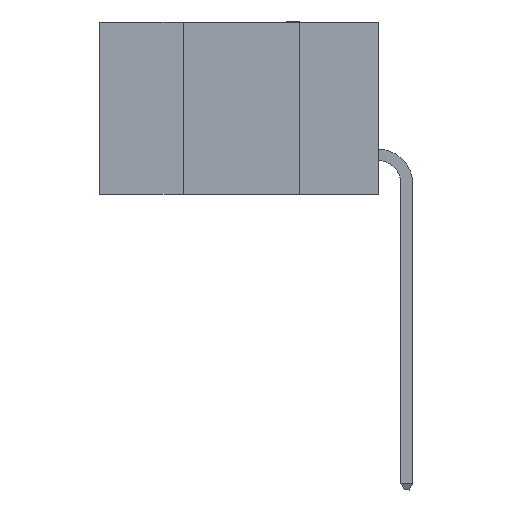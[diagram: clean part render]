
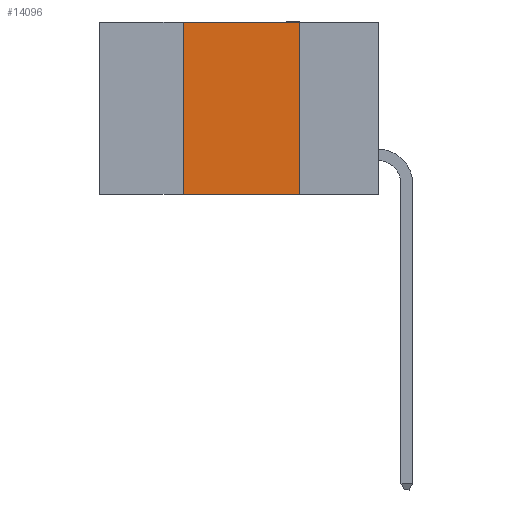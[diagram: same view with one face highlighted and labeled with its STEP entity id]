
A CAD part, left-side view. The second image highlights one B-rep face of the part: STEP entity #14096.
In plain terms, the highlighted planar face has unit normal (-1, 0, 0).
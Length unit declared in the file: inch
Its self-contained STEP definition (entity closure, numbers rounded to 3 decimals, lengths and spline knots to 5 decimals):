
#44 = EDGE_LOOP ( 'NONE', ( #13798, #10727, #9750, #3864 ) ) ;
#393 = FACE_OUTER_BOUND ( 'NONE', #44, .T. ) ;
#962 = VERTEX_POINT ( 'NONE', #5212 ) ;
#1125 = VECTOR ( 'NONE', #3401, 39.37008 ) ;
#1788 = CARTESIAN_POINT ( 'NONE',  ( 0., 0.17, 0. ) ) ;
#1897 = PLANE ( 'NONE',  #8837 ) ;
#2640 = VERTEX_POINT ( 'NONE', #10346 ) ;
#3098 = DIRECTION ( 'NONE',  ( 0., 0., -1. ) ) ;
#3101 = DIRECTION ( 'NONE',  ( 0., 0., 1. ) ) ;
#3401 = DIRECTION ( 'NONE',  ( 0., -1., 0. ) ) ;
#3864 = ORIENTED_EDGE ( 'NONE', *, *, #14314, .T. ) ;
#4632 = VECTOR ( 'NONE', #3101, 39.37008 ) ;
#4751 = DIRECTION ( 'NONE',  ( 0., -1., 0. ) ) ;
#5212 = CARTESIAN_POINT ( 'NONE',  ( 0., 0.17, -0.37 ) ) ;
#5294 = DIRECTION ( 'NONE',  ( 1., 0., 0. ) ) ;
#5387 = CARTESIAN_POINT ( 'NONE',  ( 0., 0.6, 0. ) ) ;
#5408 = LINE ( 'NONE', #10772, #12313 ) ;
#6463 = CARTESIAN_POINT ( 'NONE',  ( 0., 0.17, 0. ) ) ;
#6552 = CARTESIAN_POINT ( 'NONE',  ( 0., 0.42, 0. ) ) ;
#6623 = EDGE_CURVE ( 'NONE', #2640, #13649, #8579, .T. ) ;
#7490 = LINE ( 'NONE', #10611, #1125 ) ;
#8579 = LINE ( 'NONE', #6552, #4632 ) ;
#8610 = EDGE_CURVE ( 'NONE', #15246, #962, #10756, .T. ) ;
#8837 = AXIS2_PLACEMENT_3D ( 'NONE', #5387, #5294, #3098 ) ;
#9067 = CARTESIAN_POINT ( 'NONE',  ( 0., 0.42, 0. ) ) ;
#9750 = ORIENTED_EDGE ( 'NONE', *, *, #6623, .F. ) ;
#9994 = VECTOR ( 'NONE', #12695, 39.37008 ) ;
#10346 = CARTESIAN_POINT ( 'NONE',  ( 0., 0.42, -0.37 ) ) ;
#10611 = CARTESIAN_POINT ( 'NONE',  ( 0., 0.6, -0.37 ) ) ;
#10727 = ORIENTED_EDGE ( 'NONE', *, *, #14335, .F. ) ;
#10756 = LINE ( 'NONE', #1788, #9994 ) ;
#10772 = CARTESIAN_POINT ( 'NONE',  ( 0., 0.6, 0. ) ) ;
#12313 = VECTOR ( 'NONE', #4751, 39.37008 ) ;
#12695 = DIRECTION ( 'NONE',  ( 0., 0., -1. ) ) ;
#13649 = VERTEX_POINT ( 'NONE', #9067 ) ;
#13798 = ORIENTED_EDGE ( 'NONE', *, *, #8610, .F. ) ;
#14096 = ADVANCED_FACE ( 'NONE', ( #393 ), #1897, .F. ) ;
#14314 = EDGE_CURVE ( 'NONE', #2640, #962, #7490, .T. ) ;
#14335 = EDGE_CURVE ( 'NONE', #13649, #15246, #5408, .T. ) ;
#15246 = VERTEX_POINT ( 'NONE', #6463 ) ;
